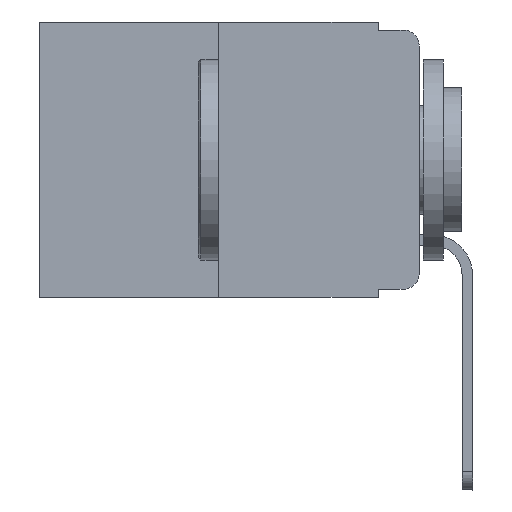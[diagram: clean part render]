
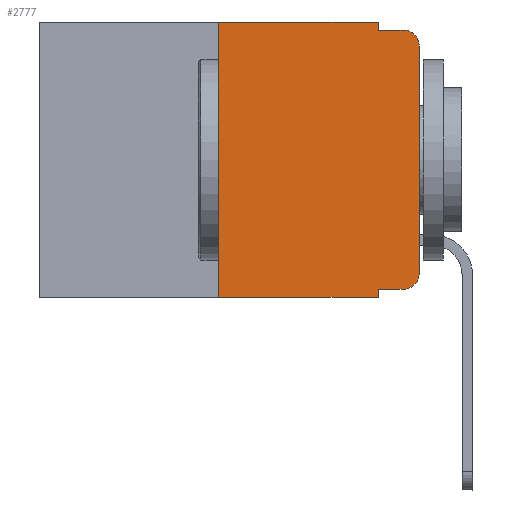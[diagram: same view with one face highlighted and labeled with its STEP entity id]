
A CAD part, left-side view. The second image highlights one B-rep face of the part: STEP entity #2777.
In plain terms, the highlighted planar face has unit normal (-1, 0, 0).
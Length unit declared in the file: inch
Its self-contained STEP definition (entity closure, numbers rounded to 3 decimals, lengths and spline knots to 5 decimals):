
#7 = AXIS2_PLACEMENT_3D ( 'NONE', #17411, #10196, #11887 ) ;
#122 = CARTESIAN_POINT ( 'NONE',  ( 0., 0., -0.313 ) ) ;
#215 = LINE ( 'NONE', #6030, #10089 ) ;
#305 = ORIENTED_EDGE ( 'NONE', *, *, #3742, .T. ) ;
#666 = DIRECTION ( 'NONE',  ( 1., 0., 0. ) ) ;
#731 = LINE ( 'NONE', #1875, #16171 ) ;
#961 = EDGE_CURVE ( 'NONE', #11020, #11857, #215, .T. ) ;
#1571 = VECTOR ( 'NONE', #1599, 39.37008 ) ;
#1599 = DIRECTION ( 'NONE',  ( 0., 0., -1. ) ) ;
#1811 = CARTESIAN_POINT ( 'NONE',  ( 0., 0.25, -0.343 ) ) ;
#1836 = LINE ( 'NONE', #11945, #12646 ) ;
#1875 = CARTESIAN_POINT ( 'NONE',  ( 0., 0., 0. ) ) ;
#2325 = CARTESIAN_POINT ( 'NONE',  ( 0., 0.051, 0. ) ) ;
#2544 = CARTESIAN_POINT ( 'NONE',  ( 0., 0.473, -0.343 ) ) ;
#2777 = ADVANCED_FACE ( 'NONE', ( #18001 ), #10774, .F. ) ;
#2885 = DIRECTION ( 'NONE',  ( 0., 0., -1. ) ) ;
#3332 = AXIS2_PLACEMENT_3D ( 'NONE', #11559, #14221, #2885 ) ;
#3525 = CARTESIAN_POINT ( 'NONE',  ( 0., 0.473, 0. ) ) ;
#3742 = EDGE_CURVE ( 'NONE', #6979, #16797, #14281, .T. ) ;
#3883 = DIRECTION ( 'NONE',  ( 0., -1., 0. ) ) ;
#3972 = CARTESIAN_POINT ( 'NONE',  ( 0., 0., -0.03 ) ) ;
#4116 = VERTEX_POINT ( 'NONE', #17331 ) ;
#4274 = VECTOR ( 'NONE', #7968, 39.37008 ) ;
#4695 = DIRECTION ( 'NONE',  ( 0., 0., -1. ) ) ;
#4763 = LINE ( 'NONE', #14962, #13838 ) ;
#4820 = ORIENTED_EDGE ( 'NONE', *, *, #11082, .T. ) ;
#5253 = CARTESIAN_POINT ( 'NONE',  ( 0., 0.02, -0.333 ) ) ;
#5426 = ORIENTED_EDGE ( 'NONE', *, *, #10623, .F. ) ;
#5876 = VERTEX_POINT ( 'NONE', #5253 ) ;
#6030 = CARTESIAN_POINT ( 'NONE',  ( 0., 0.25, 0. ) ) ;
#6337 = LINE ( 'NONE', #16514, #4274 ) ;
#6482 = DIRECTION ( 'NONE',  ( 0., 0., -1. ) ) ;
#6488 = VERTEX_POINT ( 'NONE', #7052 ) ;
#6645 = EDGE_CURVE ( 'NONE', #5876, #10497, #7933, .T. ) ;
#6917 = AXIS2_PLACEMENT_3D ( 'NONE', #3525, #666, #6482 ) ;
#6979 = VERTEX_POINT ( 'NONE', #3972 ) ;
#7033 = LINE ( 'NONE', #2544, #7236 ) ;
#7052 = CARTESIAN_POINT ( 'NONE',  ( 0., 0.051, -0.333 ) ) ;
#7236 = VECTOR ( 'NONE', #3883, 39.37008 ) ;
#7543 = EDGE_CURVE ( 'NONE', #14284, #16797, #12997, .T. ) ;
#7590 = ORIENTED_EDGE ( 'NONE', *, *, #8557, .F. ) ;
#7887 = EDGE_CURVE ( 'NONE', #9049, #14284, #10466, .T. ) ;
#7933 = CIRCLE ( 'NONE', #7, 0.02 ) ;
#7946 = CARTESIAN_POINT ( 'NONE',  ( 0., 0.25, 0. ) ) ;
#7968 = DIRECTION ( 'NONE',  ( 0., -1., 0. ) ) ;
#8078 = EDGE_CURVE ( 'NONE', #10497, #6979, #731, .T. ) ;
#8557 = EDGE_CURVE ( 'NONE', #11857, #9049, #6337, .T. ) ;
#9049 = VERTEX_POINT ( 'NONE', #2325 ) ;
#9237 = CARTESIAN_POINT ( 'NONE',  ( 0., 0.051, -0.01 ) ) ;
#9547 = DIRECTION ( 'NONE',  ( 0., -1., 0. ) ) ;
#9901 = EDGE_CURVE ( 'NONE', #11020, #4116, #7033, .T. ) ;
#10089 = VECTOR ( 'NONE', #11849, 39.37008 ) ;
#10196 = DIRECTION ( 'NONE',  ( -1., 0., 0. ) ) ;
#10466 = LINE ( 'NONE', #14842, #1571 ) ;
#10497 = VERTEX_POINT ( 'NONE', #122 ) ;
#10623 = EDGE_CURVE ( 'NONE', #6488, #4116, #1836, .T. ) ;
#10774 = PLANE ( 'NONE',  #6917 ) ;
#10942 = DIRECTION ( 'NONE',  ( 0., 0., 1. ) ) ;
#11020 = VERTEX_POINT ( 'NONE', #1811 ) ;
#11061 = ORIENTED_EDGE ( 'NONE', *, *, #961, .F. ) ;
#11082 = EDGE_CURVE ( 'NONE', #6488, #5876, #4763, .T. ) ;
#11114 = ORIENTED_EDGE ( 'NONE', *, *, #6645, .T. ) ;
#11308 = VECTOR ( 'NONE', #16124, 39.37008 ) ;
#11559 = CARTESIAN_POINT ( 'NONE',  ( 0., 0.02, -0.03 ) ) ;
#11736 = ORIENTED_EDGE ( 'NONE', *, *, #7887, .F. ) ;
#11762 = EDGE_LOOP ( 'NONE', ( #17558, #305, #14694, #11736, #7590, #11061, #17960, #5426, #4820, #11114 ) ) ;
#11849 = DIRECTION ( 'NONE',  ( 0., 0., 1. ) ) ;
#11857 = VERTEX_POINT ( 'NONE', #7946 ) ;
#11887 = DIRECTION ( 'NONE',  ( 0., 0., -1. ) ) ;
#11945 = CARTESIAN_POINT ( 'NONE',  ( 0., 0.051, 0. ) ) ;
#12304 = CARTESIAN_POINT ( 'NONE',  ( 0., 0.02, -0.01 ) ) ;
#12646 = VECTOR ( 'NONE', #4695, 39.37008 ) ;
#12997 = LINE ( 'NONE', #18799, #11308 ) ;
#13838 = VECTOR ( 'NONE', #9547, 39.37008 ) ;
#14221 = DIRECTION ( 'NONE',  ( -1., 0., 0. ) ) ;
#14281 = CIRCLE ( 'NONE', #3332, 0.02 ) ;
#14284 = VERTEX_POINT ( 'NONE', #9237 ) ;
#14694 = ORIENTED_EDGE ( 'NONE', *, *, #7543, .F. ) ;
#14842 = CARTESIAN_POINT ( 'NONE',  ( 0., 0.051, 0. ) ) ;
#14962 = CARTESIAN_POINT ( 'NONE',  ( 0., 0.051, -0.333 ) ) ;
#16124 = DIRECTION ( 'NONE',  ( 0., -1., 0. ) ) ;
#16171 = VECTOR ( 'NONE', #10942, 39.37008 ) ;
#16514 = CARTESIAN_POINT ( 'NONE',  ( 0., 0.473, 0. ) ) ;
#16797 = VERTEX_POINT ( 'NONE', #12304 ) ;
#17331 = CARTESIAN_POINT ( 'NONE',  ( 0., 0.051, -0.343 ) ) ;
#17411 = CARTESIAN_POINT ( 'NONE',  ( 0., 0.02, -0.313 ) ) ;
#17558 = ORIENTED_EDGE ( 'NONE', *, *, #8078, .T. ) ;
#17960 = ORIENTED_EDGE ( 'NONE', *, *, #9901, .T. ) ;
#18001 = FACE_OUTER_BOUND ( 'NONE', #11762, .T. ) ;
#18799 = CARTESIAN_POINT ( 'NONE',  ( 0., 0.051, -0.01 ) ) ;
